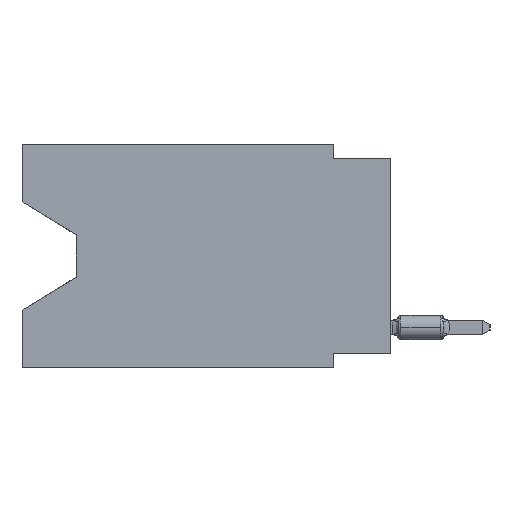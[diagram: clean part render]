
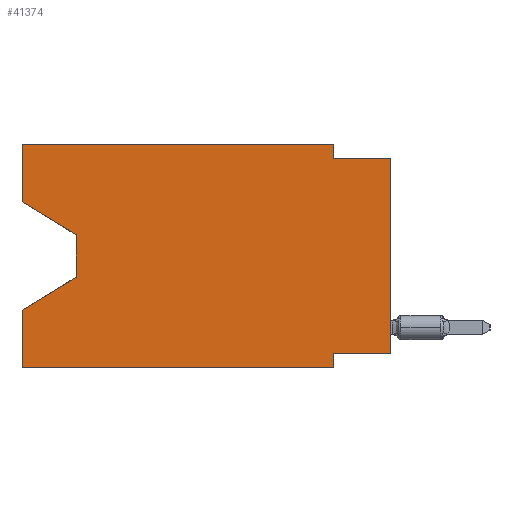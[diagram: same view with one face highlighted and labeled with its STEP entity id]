
A CAD part, left-side view. The second image highlights one B-rep face of the part: STEP entity #41374.
In plain terms, the highlighted planar face has unit normal (-1, 0, 0).
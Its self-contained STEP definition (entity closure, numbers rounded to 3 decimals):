
#2157 = CARTESIAN_POINT ( 'NONE',  ( 0., 13.97, -4.013 ) ) ;
#2229 = CARTESIAN_POINT ( 'NONE',  ( 0., 2.54, -9.271 ) ) ;
#2705 = LINE ( 'NONE', #3234, #18306 ) ;
#2884 = EDGE_CURVE ( 'NONE', #41988, #8251, #12202, .T. ) ;
#3234 = CARTESIAN_POINT ( 'NONE',  ( 0., 0., -0.635 ) ) ;
#3423 = VECTOR ( 'NONE', #3849, 1000. ) ;
#3768 = CARTESIAN_POINT ( 'NONE',  ( 0., 0., -0.635 ) ) ;
#3849 = DIRECTION ( 'NONE',  ( 0., 0., -1. ) ) ;
#4718 = ORIENTED_EDGE ( 'NONE', *, *, #33006, .T. ) ;
#5949 = ORIENTED_EDGE ( 'NONE', *, *, #47382, .F. ) ;
#6083 = DIRECTION ( 'NONE',  ( 0., 0., 1. ) ) ;
#7073 = DIRECTION ( 'NONE',  ( 0., 1., 0. ) ) ;
#7584 = LINE ( 'NONE', #27284, #46282 ) ;
#7812 = EDGE_CURVE ( 'NONE', #10886, #7965, #46987, .T. ) ;
#7836 = DIRECTION ( 'NONE',  ( 0., 0., 1. ) ) ;
#7965 = VERTEX_POINT ( 'NONE', #27725 ) ;
#8251 = VERTEX_POINT ( 'NONE', #2157 ) ;
#8478 = LINE ( 'NONE', #24690, #37600 ) ;
#9097 = AXIS2_PLACEMENT_3D ( 'NONE', #15044, #31001, #51698 ) ;
#9390 = CARTESIAN_POINT ( 'NONE',  ( 0., 16.383, -9.906 ) ) ;
#9720 = LINE ( 'NONE', #29380, #44163 ) ;
#10886 = VERTEX_POINT ( 'NONE', #2229 ) ;
#10955 = ORIENTED_EDGE ( 'NONE', *, *, #47225, .F. ) ;
#11377 = DIRECTION ( 'NONE',  ( 0., -1., 0. ) ) ;
#11563 = PLANE ( 'NONE',  #9097 ) ;
#11872 = EDGE_CURVE ( 'NONE', #35331, #39472, #9720, .T. ) ;
#11902 = VERTEX_POINT ( 'NONE', #45838 ) ;
#12202 = LINE ( 'NONE', #28164, #19948 ) ;
#12720 = CARTESIAN_POINT ( 'NONE',  ( 0., 2.54, 0. ) ) ;
#14129 = EDGE_CURVE ( 'NONE', #17007, #25805, #20058, .T. ) ;
#14428 = VECTOR ( 'NONE', #34211, 1000. ) ;
#14517 = VECTOR ( 'NONE', #11377, 1000. ) ;
#15044 = CARTESIAN_POINT ( 'NONE',  ( 0., 16.383, 0. ) ) ;
#15234 = DIRECTION ( 'NONE',  ( 0., 0.855, -0.519 ) ) ;
#16187 = ORIENTED_EDGE ( 'NONE', *, *, #7812, .F. ) ;
#17007 = VERTEX_POINT ( 'NONE', #36467 ) ;
#17428 = DIRECTION ( 'NONE',  ( 0., -1., 0. ) ) ;
#18306 = VECTOR ( 'NONE', #18387, 1000. ) ;
#18387 = DIRECTION ( 'NONE',  ( 0., -1., 0. ) ) ;
#18433 = EDGE_CURVE ( 'NONE', #39472, #38402, #8478, .T. ) ;
#19203 = ORIENTED_EDGE ( 'NONE', *, *, #11872, .F. ) ;
#19301 = FACE_OUTER_BOUND ( 'NONE', #43272, .T. ) ;
#19801 = LINE ( 'NONE', #36004, #3423 ) ;
#19948 = VECTOR ( 'NONE', #40108, 1000. ) ;
#20058 = LINE ( 'NONE', #28295, #51112 ) ;
#20791 = VECTOR ( 'NONE', #21517, 1000. ) ;
#21457 = ORIENTED_EDGE ( 'NONE', *, *, #18433, .F. ) ;
#21517 = DIRECTION ( 'NONE',  ( 0., 0., -1. ) ) ;
#21622 = VECTOR ( 'NONE', #6083, 1000. ) ;
#21747 = ORIENTED_EDGE ( 'NONE', *, *, #22190, .T. ) ;
#22190 = EDGE_CURVE ( 'NONE', #8251, #43356, #19801, .T. ) ;
#22575 = EDGE_CURVE ( 'NONE', #43356, #11902, #31199, .T. ) ;
#24145 = ORIENTED_EDGE ( 'NONE', *, *, #46593, .F. ) ;
#24661 = VECTOR ( 'NONE', #15234, 1000. ) ;
#24690 = CARTESIAN_POINT ( 'NONE',  ( 0., 2.54, 0. ) ) ;
#25332 = ORIENTED_EDGE ( 'NONE', *, *, #49347, .F. ) ;
#25447 = CARTESIAN_POINT ( 'NONE',  ( 0., 16.383, 0. ) ) ;
#25805 = VERTEX_POINT ( 'NONE', #3768 ) ;
#27284 = CARTESIAN_POINT ( 'NONE',  ( 0., 0., -9.271 ) ) ;
#27725 = CARTESIAN_POINT ( 'NONE',  ( 0., 2.54, -9.906 ) ) ;
#28164 = CARTESIAN_POINT ( 'NONE',  ( 0., 16.383, -2.546 ) ) ;
#28295 = CARTESIAN_POINT ( 'NONE',  ( 0., 0., 0. ) ) ;
#29380 = CARTESIAN_POINT ( 'NONE',  ( 0., 16.383, 0. ) ) ;
#29418 = LINE ( 'NONE', #25447, #14428 ) ;
#31001 = DIRECTION ( 'NONE',  ( 1., 0., 0. ) ) ;
#31199 = LINE ( 'NONE', #35950, #24661 ) ;
#31562 = CARTESIAN_POINT ( 'NONE',  ( 0., 2.54, -0.635 ) ) ;
#32108 = CARTESIAN_POINT ( 'NONE',  ( 0., 16.383, -9.906 ) ) ;
#33006 = EDGE_CURVE ( 'NONE', #44693, #7965, #51764, .T. ) ;
#34211 = DIRECTION ( 'NONE',  ( 0., 0., 1. ) ) ;
#34525 = ORIENTED_EDGE ( 'NONE', *, *, #2884, .T. ) ;
#35331 = VERTEX_POINT ( 'NONE', #42318 ) ;
#35950 = CARTESIAN_POINT ( 'NONE',  ( 0., 13.97, -5.893 ) ) ;
#36004 = CARTESIAN_POINT ( 'NONE',  ( 0., 13.97, -4.013 ) ) ;
#36467 = CARTESIAN_POINT ( 'NONE',  ( 0., 0., -9.271 ) ) ;
#37018 = ORIENTED_EDGE ( 'NONE', *, *, #14129, .T. ) ;
#37600 = VECTOR ( 'NONE', #40882, 1000. ) ;
#38402 = VERTEX_POINT ( 'NONE', #31562 ) ;
#39472 = VERTEX_POINT ( 'NONE', #12720 ) ;
#40108 = DIRECTION ( 'NONE',  ( 0., -0.855, -0.519 ) ) ;
#40882 = DIRECTION ( 'NONE',  ( 0., 0., -1. ) ) ;
#41374 = ADVANCED_FACE ( 'NONE', ( #19301 ), #11563, .F. ) ;
#41693 = CARTESIAN_POINT ( 'NONE',  ( 0., 16.383, 0. ) ) ;
#41988 = VERTEX_POINT ( 'NONE', #48418 ) ;
#42318 = CARTESIAN_POINT ( 'NONE',  ( 0., 16.383, 0. ) ) ;
#43272 = EDGE_LOOP ( 'NONE', ( #34525, #21747, #45511, #24145, #4718, #16187, #10955, #37018, #5949, #21457, #19203, #25332 ) ) ;
#43356 = VERTEX_POINT ( 'NONE', #50337 ) ;
#44163 = VECTOR ( 'NONE', #17428, 1000. ) ;
#44693 = VERTEX_POINT ( 'NONE', #9390 ) ;
#45135 = LINE ( 'NONE', #41693, #21622 ) ;
#45511 = ORIENTED_EDGE ( 'NONE', *, *, #22575, .T. ) ;
#45838 = CARTESIAN_POINT ( 'NONE',  ( 0., 16.383, -7.36 ) ) ;
#46282 = VECTOR ( 'NONE', #7073, 1000. ) ;
#46593 = EDGE_CURVE ( 'NONE', #44693, #11902, #45135, .T. ) ;
#46987 = LINE ( 'NONE', #50711, #20791 ) ;
#47225 = EDGE_CURVE ( 'NONE', #17007, #10886, #7584, .T. ) ;
#47382 = EDGE_CURVE ( 'NONE', #38402, #25805, #2705, .T. ) ;
#48418 = CARTESIAN_POINT ( 'NONE',  ( 0., 16.383, -2.546 ) ) ;
#49347 = EDGE_CURVE ( 'NONE', #41988, #35331, #29418, .T. ) ;
#50337 = CARTESIAN_POINT ( 'NONE',  ( 0., 13.97, -5.893 ) ) ;
#50711 = CARTESIAN_POINT ( 'NONE',  ( 0., 2.54, -9.906 ) ) ;
#51112 = VECTOR ( 'NONE', #7836, 1000. ) ;
#51698 = DIRECTION ( 'NONE',  ( 0., 0., -1. ) ) ;
#51764 = LINE ( 'NONE', #32108, #14517 ) ;
